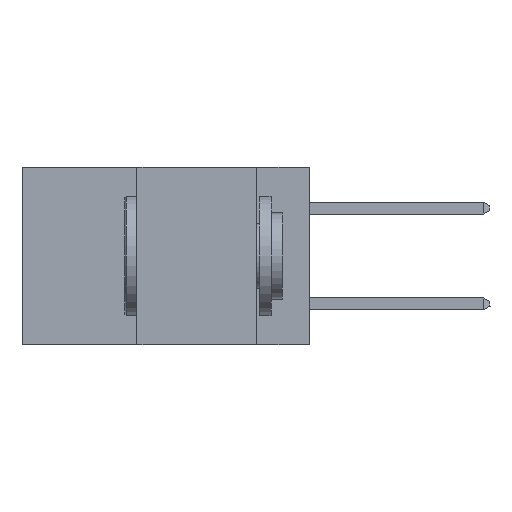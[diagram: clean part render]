
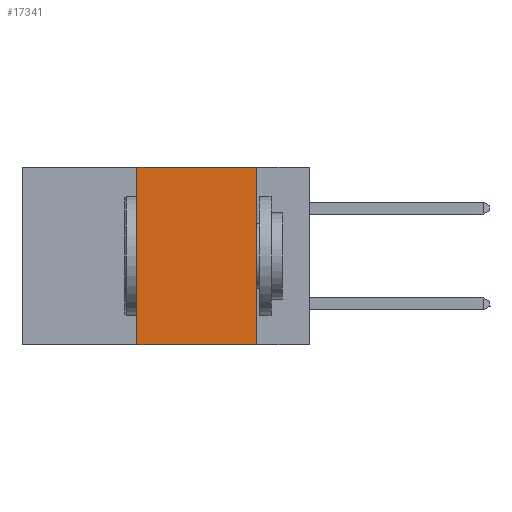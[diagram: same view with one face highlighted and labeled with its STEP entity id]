
A CAD part, left-side view. The second image highlights one B-rep face of the part: STEP entity #17341.
In plain terms, the highlighted planar face has unit normal (-1, 0, 0).
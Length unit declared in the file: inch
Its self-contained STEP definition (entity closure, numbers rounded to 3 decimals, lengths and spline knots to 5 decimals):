
#199 = EDGE_CURVE ( 'NONE', #222, #22634, #25767, .T. ) ;
#222 = VERTEX_POINT ( 'NONE', #23635 ) ;
#549 = CARTESIAN_POINT ( 'NONE',  ( 0., 0.11, 0. ) ) ;
#1949 = CARTESIAN_POINT ( 'NONE',  ( 0., 0.6, -0.37 ) ) ;
#2018 = VERTEX_POINT ( 'NONE', #16433 ) ;
#3573 = LINE ( 'NONE', #549, #23219 ) ;
#4528 = EDGE_CURVE ( 'NONE', #5072, #2018, #7694, .T. ) ;
#4741 = EDGE_CURVE ( 'NONE', #5072, #222, #17970, .T. ) ;
#5072 = VERTEX_POINT ( 'NONE', #11308 ) ;
#5107 = DIRECTION ( 'NONE',  ( 0., -1., 0. ) ) ;
#5658 = DIRECTION ( 'NONE',  ( 0., 0., -1. ) ) ;
#6533 = ORIENTED_EDGE ( 'NONE', *, *, #4741, .F. ) ;
#7245 = CARTESIAN_POINT ( 'NONE',  ( 0., 0.11, 0. ) ) ;
#7416 = AXIS2_PLACEMENT_3D ( 'NONE', #17993, #21945, #5658 ) ;
#7694 = LINE ( 'NONE', #1949, #15340 ) ;
#8204 = ORIENTED_EDGE ( 'NONE', *, *, #199, .F. ) ;
#8851 = EDGE_LOOP ( 'NONE', ( #15241, #8204, #6533, #16043 ) ) ;
#11308 = CARTESIAN_POINT ( 'NONE',  ( 0., 0.36, -0.37 ) ) ;
#13343 = DIRECTION ( 'NONE',  ( 0., 0., 1. ) ) ;
#14119 = FACE_OUTER_BOUND ( 'NONE', #8851, .T. ) ;
#15241 = ORIENTED_EDGE ( 'NONE', *, *, #18810, .F. ) ;
#15340 = VECTOR ( 'NONE', #22574, 39.37008 ) ;
#15580 = CARTESIAN_POINT ( 'NONE',  ( 0., 0.6, 0. ) ) ;
#15964 = PLANE ( 'NONE',  #7416 ) ;
#16043 = ORIENTED_EDGE ( 'NONE', *, *, #4528, .T. ) ;
#16433 = CARTESIAN_POINT ( 'NONE',  ( 0., 0.11, -0.37 ) ) ;
#17341 = ADVANCED_FACE ( 'NONE', ( #14119 ), #15964, .F. ) ;
#17970 = LINE ( 'NONE', #21279, #20859 ) ;
#17993 = CARTESIAN_POINT ( 'NONE',  ( 0., 0.6, 0. ) ) ;
#18810 = EDGE_CURVE ( 'NONE', #22634, #2018, #3573, .T. ) ;
#20326 = VECTOR ( 'NONE', #5107, 39.37008 ) ;
#20859 = VECTOR ( 'NONE', #13343, 39.37008 ) ;
#21279 = CARTESIAN_POINT ( 'NONE',  ( 0., 0.36, 0. ) ) ;
#21945 = DIRECTION ( 'NONE',  ( 1., 0., 0. ) ) ;
#22574 = DIRECTION ( 'NONE',  ( 0., -1., 0. ) ) ;
#22634 = VERTEX_POINT ( 'NONE', #7245 ) ;
#22939 = DIRECTION ( 'NONE',  ( 0., 0., -1. ) ) ;
#23219 = VECTOR ( 'NONE', #22939, 39.37008 ) ;
#23635 = CARTESIAN_POINT ( 'NONE',  ( 0., 0.36, 0. ) ) ;
#25767 = LINE ( 'NONE', #15580, #20326 ) ;
